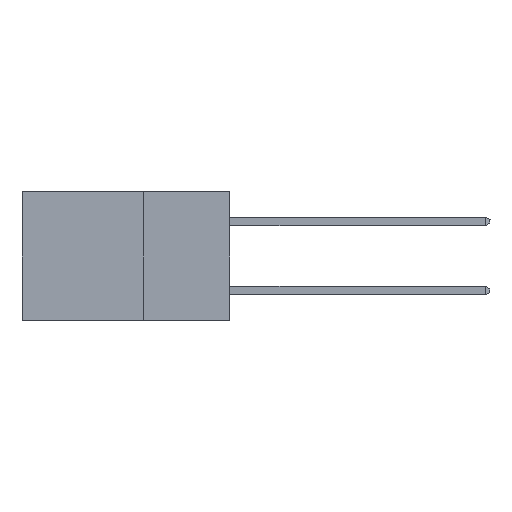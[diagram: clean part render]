
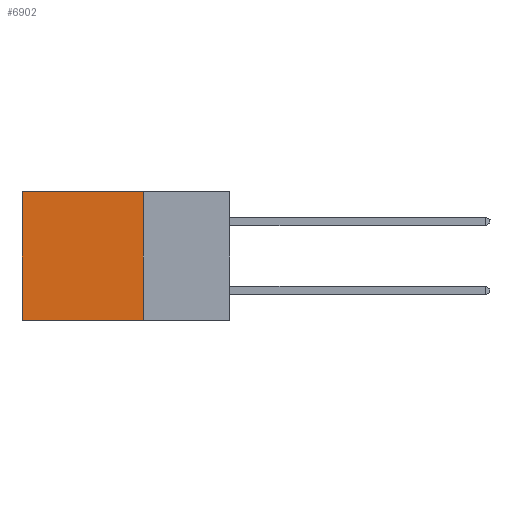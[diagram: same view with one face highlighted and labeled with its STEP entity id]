
A CAD part, left-side view. The second image highlights one B-rep face of the part: STEP entity #6902.
In plain terms, the highlighted planar face has unit normal (-1, 0, 0).
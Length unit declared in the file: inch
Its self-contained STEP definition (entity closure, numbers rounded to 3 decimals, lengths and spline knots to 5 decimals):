
#406 = VECTOR ( 'NONE', #8269, 39.37008 ) ;
#623 = LINE ( 'NONE', #16392, #5190 ) ;
#1763 = CARTESIAN_POINT ( 'NONE',  ( 0.2615, 0.25, -0.37 ) ) ;
#4866 = EDGE_CURVE ( 'NONE', #14854, #8115, #6271, .T. ) ;
#5190 = VECTOR ( 'NONE', #12164, 39.37008 ) ;
#6271 = LINE ( 'NONE', #17767, #12539 ) ;
#6669 = VECTOR ( 'NONE', #12251, 39.37008 ) ;
#6902 = ADVANCED_FACE ( 'NONE', ( #11503 ), #14705, .F. ) ;
#7016 = VERTEX_POINT ( 'NONE', #7335 ) ;
#7202 = EDGE_CURVE ( 'NONE', #15142, #8115, #10645, .T. ) ;
#7335 = CARTESIAN_POINT ( 'NONE',  ( 0.2615, 0.25, 0. ) ) ;
#7903 = CARTESIAN_POINT ( 'NONE',  ( 0.2615, 0.6, -0.37 ) ) ;
#8115 = VERTEX_POINT ( 'NONE', #18565 ) ;
#8269 = DIRECTION ( 'NONE',  ( 0., 0., -1. ) ) ;
#8768 = DIRECTION ( 'NONE',  ( 0., 0., -1. ) ) ;
#10078 = DIRECTION ( 'NONE',  ( 1., 0., 0. ) ) ;
#10617 = DIRECTION ( 'NONE',  ( 0., 1., 0. ) ) ;
#10645 = LINE ( 'NONE', #7903, #6669 ) ;
#10723 = CARTESIAN_POINT ( 'NONE',  ( 0.2615, 0.6, 0. ) ) ;
#11503 = FACE_OUTER_BOUND ( 'NONE', #11707, .T. ) ;
#11707 = EDGE_LOOP ( 'NONE', ( #12633, #16191, #16486, #18004 ) ) ;
#12164 = DIRECTION ( 'NONE',  ( 0., 1., 0. ) ) ;
#12251 = DIRECTION ( 'NONE',  ( 0., 0., -1. ) ) ;
#12539 = VECTOR ( 'NONE', #10617, 39.37008 ) ;
#12633 = ORIENTED_EDGE ( 'NONE', *, *, #7202, .T. ) ;
#14705 = PLANE ( 'NONE',  #16896 ) ;
#14854 = VERTEX_POINT ( 'NONE', #17596 ) ;
#15142 = VERTEX_POINT ( 'NONE', #10723 ) ;
#15695 = CARTESIAN_POINT ( 'NONE',  ( 0.2615, 0.25, -0.37 ) ) ;
#15983 = EDGE_CURVE ( 'NONE', #7016, #15142, #623, .T. ) ;
#16191 = ORIENTED_EDGE ( 'NONE', *, *, #4866, .F. ) ;
#16392 = CARTESIAN_POINT ( 'NONE',  ( 0.2615, 0.25, 0. ) ) ;
#16486 = ORIENTED_EDGE ( 'NONE', *, *, #18083, .F. ) ;
#16896 = AXIS2_PLACEMENT_3D ( 'NONE', #1763, #10078, #8768 ) ;
#17596 = CARTESIAN_POINT ( 'NONE',  ( 0.2615, 0.25, -0.37 ) ) ;
#17767 = CARTESIAN_POINT ( 'NONE',  ( 0.2615, 0.25, -0.37 ) ) ;
#18004 = ORIENTED_EDGE ( 'NONE', *, *, #15983, .T. ) ;
#18083 = EDGE_CURVE ( 'NONE', #7016, #14854, #18424, .T. ) ;
#18424 = LINE ( 'NONE', #15695, #406 ) ;
#18565 = CARTESIAN_POINT ( 'NONE',  ( 0.2615, 0.6, -0.37 ) ) ;
